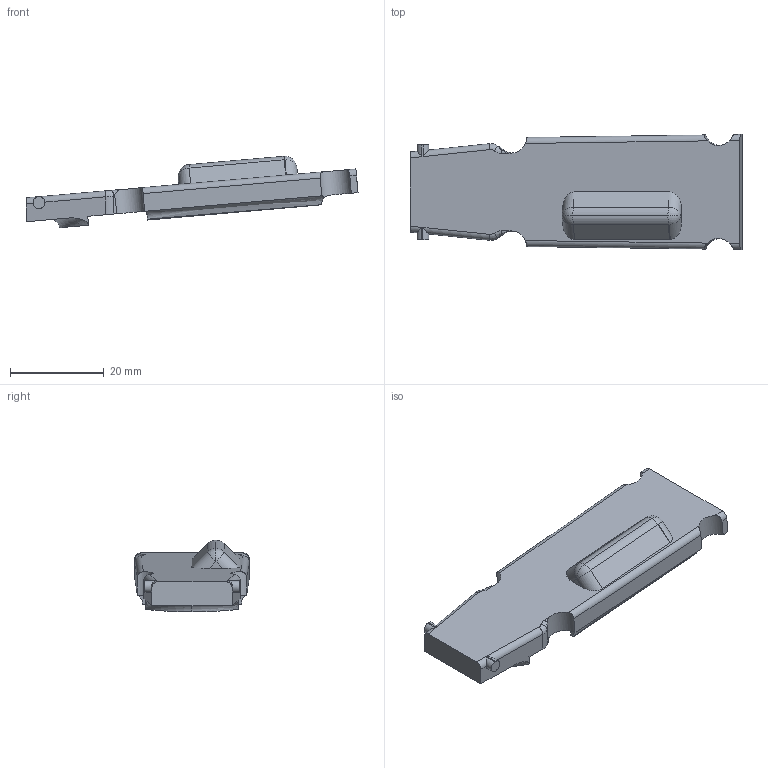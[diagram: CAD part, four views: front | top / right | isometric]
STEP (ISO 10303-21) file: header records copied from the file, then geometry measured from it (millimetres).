
FILE_DESCRIPTION (( 'STEP AP214' ), '1' );
FILE_NAME ('Follower V2.STEP', '2013-06-18T15:19:04', ( 'Asher' ), ( '' ), 'SwSTEP 2.0', 'SolidWorks 2013', '' );
FILE_SCHEMA (( 'AUTOMOTIVE_DESIGN' ));
Length unit declared in the file: millimetre
Products named in the file (1): Follower V2
Bounding box: 70.71 x 24.51 x 15.23 mm (x, y, z)
Volume: 8628.8 mm3; surface area: 4471.7 mm2
Topology: 1 solids, 1 shells, 75 faces, 201 edges, 129 vertices
Faces by surface type: cylinder 30, plane 30, bspline 9, sphere 4, torus 2
Entity records: 2697 total; most frequent: CARTESIAN_POINT 951, ORIENTED_EDGE 402, DIRECTION 309, EDGE_CURVE 201, VERTEX_POINT 129, AXIS2_PLACEMENT_3D 107, LINE 95, VECTOR 95
